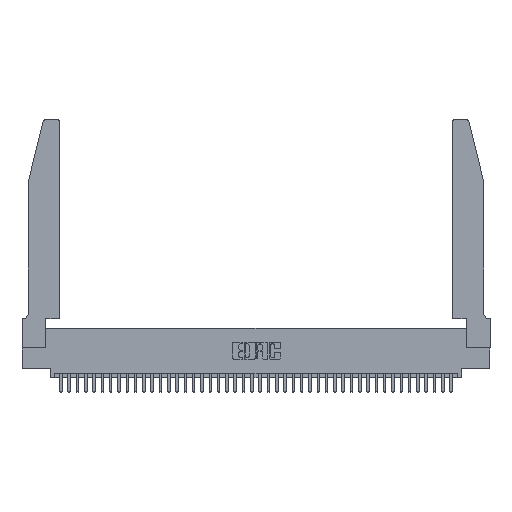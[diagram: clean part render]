
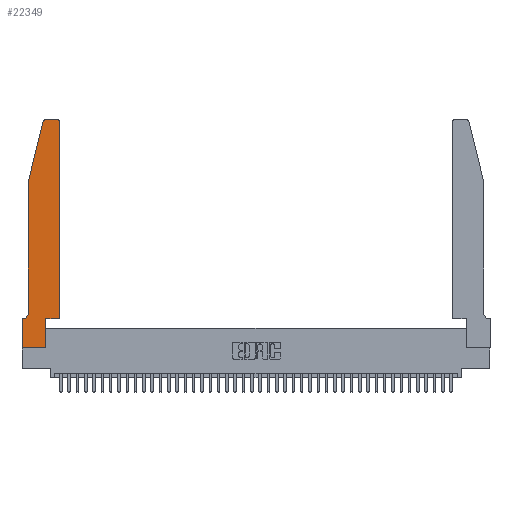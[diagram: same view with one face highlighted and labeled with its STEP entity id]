
A CAD part, top view. The second image highlights one B-rep face of the part: STEP entity #22349.
In plain terms, the highlighted planar face has unit normal (0, 0, 1).
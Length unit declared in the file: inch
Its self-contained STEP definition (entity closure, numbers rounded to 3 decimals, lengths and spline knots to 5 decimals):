
#773 = CARTESIAN_POINT ( 'NONE',  ( 0.0755, 0.35, 0.37 ) ) ;
#1613 = LINE ( 'NONE', #12520, #34989 ) ;
#2005 = VECTOR ( 'NONE', #32659, 39.37008 ) ;
#2899 = DIRECTION ( 'NONE',  ( 1., 0., 0. ) ) ;
#4104 = VERTEX_POINT ( 'NONE', #39314 ) ;
#4605 = ORIENTED_EDGE ( 'NONE', *, *, #6335, .T. ) ;
#5845 = AXIS2_PLACEMENT_3D ( 'NONE', #6684, #32586, #19543 ) ;
#6335 = EDGE_CURVE ( 'NONE', #26009, #30781, #27912, .T. ) ;
#6684 = CARTESIAN_POINT ( 'NONE',  ( 0.0055, 0.42, 0.37 ) ) ;
#6868 = VECTOR ( 'NONE', #34775, 39.37008 ) ;
#7757 = FACE_OUTER_BOUND ( 'NONE', #28883, .T. ) ;
#7809 = VERTEX_POINT ( 'NONE', #26192 ) ;
#8009 = CARTESIAN_POINT ( 'NONE',  ( 0.284, 2.72, 0.37 ) ) ;
#8140 = DIRECTION ( 'NONE',  ( 1., 0., 0. ) ) ;
#8806 = VERTEX_POINT ( 'NONE', #16099 ) ;
#9196 = CARTESIAN_POINT ( 'NONE',  ( 0., 0., 0.37 ) ) ;
#9832 = DIRECTION ( 'NONE',  ( 0., 1., 0. ) ) ;
#10228 = DIRECTION ( 'NONE',  ( -1., 0., 0. ) ) ;
#10562 = VERTEX_POINT ( 'NONE', #28521 ) ;
#11073 = CARTESIAN_POINT ( 'NONE',  ( 0.0755, 2., 0.37 ) ) ;
#11959 = PLANE ( 'NONE',  #20641 ) ;
#12315 = DIRECTION ( 'NONE',  ( 0., -1., 0. ) ) ;
#12426 = EDGE_CURVE ( 'NONE', #23629, #39271, #14835, .T. ) ;
#12520 = CARTESIAN_POINT ( 'NONE',  ( 0.2865, 0.35, 0.37 ) ) ;
#12621 = LINE ( 'NONE', #38584, #2005 ) ;
#14528 = LINE ( 'NONE', #9196, #18063 ) ;
#14835 = LINE ( 'NONE', #24310, #20362 ) ;
#16099 = CARTESIAN_POINT ( 'NONE',  ( 0., 0., 0.37 ) ) ;
#16848 = EDGE_CURVE ( 'NONE', #4104, #37425, #12621, .T. ) ;
#17518 = EDGE_CURVE ( 'NONE', #8806, #40696, #30259, .T. ) ;
#17813 = VECTOR ( 'NONE', #9832, 39.37008 ) ;
#18026 = DIRECTION ( 'NONE',  ( 0., 0., 1. ) ) ;
#18063 = VECTOR ( 'NONE', #12315, 39.37008 ) ;
#19113 = EDGE_CURVE ( 'NONE', #39223, #8806, #14528, .T. ) ;
#19118 = DIRECTION ( 'NONE',  ( 0., 0., 1. ) ) ;
#19543 = DIRECTION ( 'NONE',  ( -1., 0., 0. ) ) ;
#19562 = CARTESIAN_POINT ( 'NONE',  ( 0.4505, 0.35, 0.37 ) ) ;
#20362 = VECTOR ( 'NONE', #27456, 39.37008 ) ;
#20641 = AXIS2_PLACEMENT_3D ( 'NONE', #28169, #19118, #41776 ) ;
#21342 = ORIENTED_EDGE ( 'NONE', *, *, #33093, .T. ) ;
#21921 = ORIENTED_EDGE ( 'NONE', *, *, #19113, .T. ) ;
#22160 = ORIENTED_EDGE ( 'NONE', *, *, #40150, .T. ) ;
#22189 = EDGE_CURVE ( 'NONE', #39271, #26009, #41148, .T. ) ;
#22221 = CARTESIAN_POINT ( 'NONE',  ( 0., 0.35, 0.37 ) ) ;
#22349 = ADVANCED_FACE ( 'NONE', ( #7757 ), #11959, .T. ) ;
#22719 = ORIENTED_EDGE ( 'NONE', *, *, #41133, .T. ) ;
#22854 = LINE ( 'NONE', #19562, #17813 ) ;
#22863 = VECTOR ( 'NONE', #40353, 39.37008 ) ;
#22950 = VECTOR ( 'NONE', #10228, 39.37008 ) ;
#23629 = VERTEX_POINT ( 'NONE', #35731 ) ;
#24310 = CARTESIAN_POINT ( 'NONE',  ( 0.2605, 2.75, 0.37 ) ) ;
#24701 = CARTESIAN_POINT ( 'NONE',  ( 0.0055, 0.35, 0.37 ) ) ;
#25084 = CIRCLE ( 'NONE', #5845, 0.07 ) ;
#25124 = CARTESIAN_POINT ( 'NONE',  ( 0.4205, 2.72, 0.37 ) ) ;
#25635 = ORIENTED_EDGE ( 'NONE', *, *, #32282, .T. ) ;
#25675 = ORIENTED_EDGE ( 'NONE', *, *, #17518, .T. ) ;
#25968 = CIRCLE ( 'NONE', #31480, 0.03 ) ;
#26009 = VERTEX_POINT ( 'NONE', #30620 ) ;
#26192 = CARTESIAN_POINT ( 'NONE',  ( 0.0755, 0.42, 0.37 ) ) ;
#26442 = EDGE_CURVE ( 'NONE', #7809, #30060, #25084, .T. ) ;
#27097 = LINE ( 'NONE', #38151, #6868 ) ;
#27456 = DIRECTION ( 'NONE',  ( -1., 0., 0. ) ) ;
#27858 = ORIENTED_EDGE ( 'NONE', *, *, #35478, .T. ) ;
#27912 = LINE ( 'NONE', #11073, #22863 ) ;
#28169 = CARTESIAN_POINT ( 'NONE',  ( 0., 0.35, 0.37 ) ) ;
#28521 = CARTESIAN_POINT ( 'NONE',  ( 0.4505, 2.72, 0.37 ) ) ;
#28883 = EDGE_LOOP ( 'NONE', ( #40210, #29105, #4605, #22160, #39892, #22719, #21921, #25675, #27858, #39120, #21342, #25635 ) ) ;
#29105 = ORIENTED_EDGE ( 'NONE', *, *, #22189, .T. ) ;
#30060 = VERTEX_POINT ( 'NONE', #24701 ) ;
#30259 = LINE ( 'NONE', #41242, #40398 ) ;
#30620 = CARTESIAN_POINT ( 'NONE',  ( 0.25487, 2.72718, 0.37 ) ) ;
#30781 = VERTEX_POINT ( 'NONE', #31258 ) ;
#31258 = CARTESIAN_POINT ( 'NONE',  ( 0.0755, 2., 0.37 ) ) ;
#31480 = AXIS2_PLACEMENT_3D ( 'NONE', #25124, #34923, #38432 ) ;
#31584 = LINE ( 'NONE', #773, #22950 ) ;
#31727 = CARTESIAN_POINT ( 'NONE',  ( 0.284, 2.75, 0.37 ) ) ;
#32282 = EDGE_CURVE ( 'NONE', #10562, #23629, #25968, .T. ) ;
#32586 = DIRECTION ( 'NONE',  ( 0., 0., -1. ) ) ;
#32659 = DIRECTION ( 'NONE',  ( 1., 0., 0. ) ) ;
#33093 = EDGE_CURVE ( 'NONE', #37425, #10562, #22854, .T. ) ;
#34775 = DIRECTION ( 'NONE',  ( 0., -1., 0. ) ) ;
#34923 = DIRECTION ( 'NONE',  ( 0., 0., 1. ) ) ;
#34989 = VECTOR ( 'NONE', #41512, 39.37008 ) ;
#35478 = EDGE_CURVE ( 'NONE', #40696, #4104, #1613, .T. ) ;
#35731 = CARTESIAN_POINT ( 'NONE',  ( 0.4205, 2.75, 0.37 ) ) ;
#37425 = VERTEX_POINT ( 'NONE', #39452 ) ;
#37811 = CARTESIAN_POINT ( 'NONE',  ( 0.2865, 0., 0.37 ) ) ;
#38151 = CARTESIAN_POINT ( 'NONE',  ( 0.0755, 2., 0.37 ) ) ;
#38254 = AXIS2_PLACEMENT_3D ( 'NONE', #8009, #18026, #8140 ) ;
#38432 = DIRECTION ( 'NONE',  ( 1., 0., 0. ) ) ;
#38584 = CARTESIAN_POINT ( 'NONE',  ( 0.4505, 0.35, 0.37 ) ) ;
#39120 = ORIENTED_EDGE ( 'NONE', *, *, #16848, .T. ) ;
#39223 = VERTEX_POINT ( 'NONE', #22221 ) ;
#39271 = VERTEX_POINT ( 'NONE', #31727 ) ;
#39314 = CARTESIAN_POINT ( 'NONE',  ( 0.2865, 0.35, 0.37 ) ) ;
#39452 = CARTESIAN_POINT ( 'NONE',  ( 0.4505, 0.35, 0.37 ) ) ;
#39892 = ORIENTED_EDGE ( 'NONE', *, *, #26442, .T. ) ;
#40150 = EDGE_CURVE ( 'NONE', #30781, #7809, #27097, .T. ) ;
#40210 = ORIENTED_EDGE ( 'NONE', *, *, #12426, .T. ) ;
#40353 = DIRECTION ( 'NONE',  ( -0.239, -0.971, 0. ) ) ;
#40398 = VECTOR ( 'NONE', #2899, 39.37008 ) ;
#40696 = VERTEX_POINT ( 'NONE', #37811 ) ;
#41133 = EDGE_CURVE ( 'NONE', #30060, #39223, #31584, .T. ) ;
#41148 = CIRCLE ( 'NONE', #38254, 0.03 ) ;
#41242 = CARTESIAN_POINT ( 'NONE',  ( 0., 0., 0.37 ) ) ;
#41512 = DIRECTION ( 'NONE',  ( 0., 1., 0. ) ) ;
#41776 = DIRECTION ( 'NONE',  ( 1., 0., 0. ) ) ;
